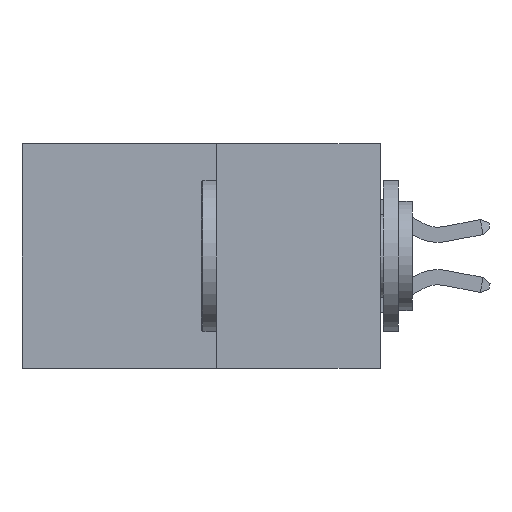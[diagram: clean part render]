
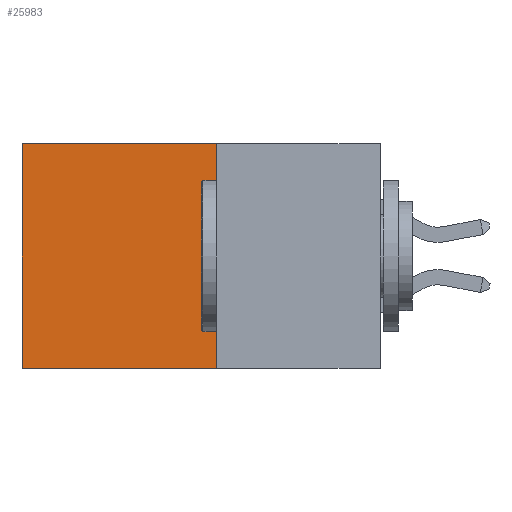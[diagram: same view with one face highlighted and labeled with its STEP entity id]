
A CAD part, left-side view. The second image highlights one B-rep face of the part: STEP entity #25983.
In plain terms, the highlighted planar face has unit normal (-1, 0, 0).
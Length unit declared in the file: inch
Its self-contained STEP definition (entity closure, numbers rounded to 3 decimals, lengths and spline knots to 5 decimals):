
#175 = ORIENTED_EDGE ( 'NONE', *, *, #20797, .T. ) ;
#871 = PLANE ( 'NONE',  #8441 ) ;
#963 = CARTESIAN_POINT ( 'NONE',  ( 0.277, 0.27, -0.37 ) ) ;
#1107 = DIRECTION ( 'NONE',  ( 0., 0., -1. ) ) ;
#1206 = EDGE_LOOP ( 'NONE', ( #7866, #10090, #5649, #175 ) ) ;
#1755 = VECTOR ( 'NONE', #6913, 39.37008 ) ;
#1763 = VECTOR ( 'NONE', #1107, 39.37008 ) ;
#2277 = LINE ( 'NONE', #16726, #18133 ) ;
#3140 = DIRECTION ( 'NONE',  ( 0., 0., -1. ) ) ;
#4151 = VECTOR ( 'NONE', #21827, 39.37008 ) ;
#5649 = ORIENTED_EDGE ( 'NONE', *, *, #8381, .F. ) ;
#6913 = DIRECTION ( 'NONE',  ( 0., 0., -1. ) ) ;
#7866 = ORIENTED_EDGE ( 'NONE', *, *, #24759, .T. ) ;
#7973 = VERTEX_POINT ( 'NONE', #26976 ) ;
#8158 = DIRECTION ( 'NONE',  ( 0., 1., 0. ) ) ;
#8381 = EDGE_CURVE ( 'NONE', #7973, #11283, #25317, .T. ) ;
#8441 = AXIS2_PLACEMENT_3D ( 'NONE', #963, #16093, #3140 ) ;
#8872 = VERTEX_POINT ( 'NONE', #12838 ) ;
#10090 = ORIENTED_EDGE ( 'NONE', *, *, #21872, .F. ) ;
#11283 = VERTEX_POINT ( 'NONE', #18868 ) ;
#12838 = CARTESIAN_POINT ( 'NONE',  ( 0.277, 0.59, -0.37 ) ) ;
#15379 = CARTESIAN_POINT ( 'NONE',  ( 0.277, 0.27, 0. ) ) ;
#15513 = CARTESIAN_POINT ( 'NONE',  ( 0.277, 0.27, -0.37 ) ) ;
#15954 = CARTESIAN_POINT ( 'NONE',  ( 0.277, 0.59, 0. ) ) ;
#16093 = DIRECTION ( 'NONE',  ( 1., 0., 0. ) ) ;
#16726 = CARTESIAN_POINT ( 'NONE',  ( 0.277, 0.27, -0.37 ) ) ;
#18133 = VECTOR ( 'NONE', #8158, 39.37008 ) ;
#18868 = CARTESIAN_POINT ( 'NONE',  ( 0.277, 0.27, -0.37 ) ) ;
#20797 = EDGE_CURVE ( 'NONE', #7973, #22308, #26300, .T. ) ;
#21827 = DIRECTION ( 'NONE',  ( 0., 1., 0. ) ) ;
#21872 = EDGE_CURVE ( 'NONE', #11283, #8872, #2277, .T. ) ;
#21954 = FACE_OUTER_BOUND ( 'NONE', #1206, .T. ) ;
#22308 = VERTEX_POINT ( 'NONE', #15954 ) ;
#24648 = LINE ( 'NONE', #26928, #1763 ) ;
#24759 = EDGE_CURVE ( 'NONE', #22308, #8872, #24648, .T. ) ;
#25317 = LINE ( 'NONE', #15513, #1755 ) ;
#25983 = ADVANCED_FACE ( 'NONE', ( #21954 ), #871, .F. ) ;
#26300 = LINE ( 'NONE', #15379, #4151 ) ;
#26928 = CARTESIAN_POINT ( 'NONE',  ( 0.277, 0.59, -0.37 ) ) ;
#26976 = CARTESIAN_POINT ( 'NONE',  ( 0.277, 0.27, 0. ) ) ;
